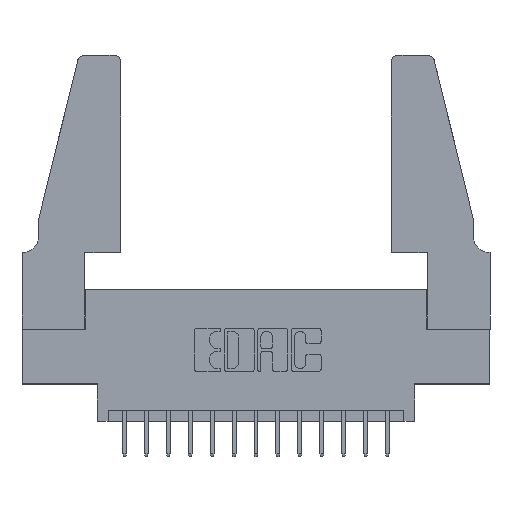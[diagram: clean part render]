
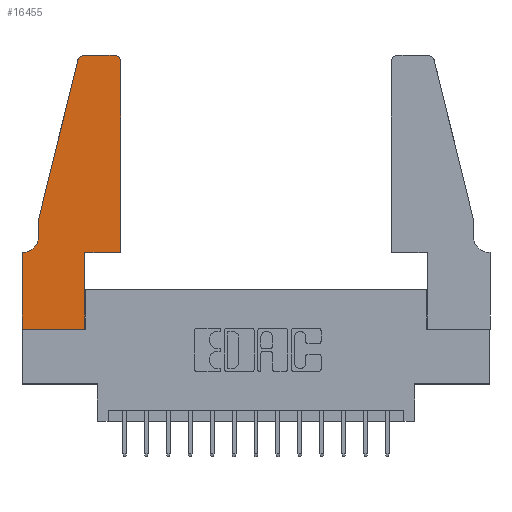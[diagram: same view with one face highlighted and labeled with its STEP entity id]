
A CAD part, top view. The second image highlights one B-rep face of the part: STEP entity #16455.
In plain terms, the highlighted planar face has unit normal (0, 0, 1).
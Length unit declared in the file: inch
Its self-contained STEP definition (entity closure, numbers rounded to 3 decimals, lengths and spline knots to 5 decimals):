
#24 = CARTESIAN_POINT ( 'NONE',  ( 0.0755, 0.5, 0.37 ) ) ;
#61 = CARTESIAN_POINT ( 'NONE',  ( 0.284, 1.25, 0.37 ) ) ;
#495 = ORIENTED_EDGE ( 'NONE', *, *, #12452, .T. ) ;
#755 = CARTESIAN_POINT ( 'NONE',  ( 0.2865, 0., 0.37 ) ) ;
#765 = CARTESIAN_POINT ( 'NONE',  ( 0.0755, 0.5, 0.37 ) ) ;
#875 = VERTEX_POINT ( 'NONE', #9621 ) ;
#919 = VECTOR ( 'NONE', #1364, 39.37008 ) ;
#1268 = ORIENTED_EDGE ( 'NONE', *, *, #7917, .T. ) ;
#1325 = VECTOR ( 'NONE', #1916, 39.37008 ) ;
#1364 = DIRECTION ( 'NONE',  ( -0.239, -0.971, 0. ) ) ;
#1634 = VECTOR ( 'NONE', #3350, 39.37008 ) ;
#1874 = CIRCLE ( 'NONE', #6621, 0.03 ) ;
#1916 = DIRECTION ( 'NONE',  ( 1., 0., 0. ) ) ;
#1967 = CARTESIAN_POINT ( 'NONE',  ( 0., 0., 0.37 ) ) ;
#2182 = ORIENTED_EDGE ( 'NONE', *, *, #4784, .T. ) ;
#2227 = VECTOR ( 'NONE', #13800, 39.37008 ) ;
#2240 = DIRECTION ( 'NONE',  ( 0., 0., 1. ) ) ;
#2303 = VERTEX_POINT ( 'NONE', #6227 ) ;
#2391 = LINE ( 'NONE', #16408, #8820 ) ;
#2397 = CARTESIAN_POINT ( 'NONE',  ( 0.4505, 1.22, 0.37 ) ) ;
#2732 = CARTESIAN_POINT ( 'NONE',  ( 0.4505, 0.35, 0.37 ) ) ;
#2824 = VERTEX_POINT ( 'NONE', #12180 ) ;
#2920 = EDGE_CURVE ( 'NONE', #9655, #12077, #4256, .T. ) ;
#3118 = PLANE ( 'NONE',  #6159 ) ;
#3288 = EDGE_CURVE ( 'NONE', #2824, #10259, #14769, .T. ) ;
#3350 = DIRECTION ( 'NONE',  ( -1., 0., 0. ) ) ;
#3437 = ORIENTED_EDGE ( 'NONE', *, *, #3288, .T. ) ;
#3443 = CARTESIAN_POINT ( 'NONE',  ( 0.0755, 0.35, 0.37 ) ) ;
#3829 = ORIENTED_EDGE ( 'NONE', *, *, #7589, .T. ) ;
#3847 = EDGE_CURVE ( 'NONE', #9854, #9655, #5633, .T. ) ;
#4188 = CARTESIAN_POINT ( 'NONE',  ( 0., 0., 0.37 ) ) ;
#4256 = CIRCLE ( 'NONE', #9482, 0.03 ) ;
#4360 = ORIENTED_EDGE ( 'NONE', *, *, #8823, .T. ) ;
#4362 = DIRECTION ( 'NONE',  ( -1., 0., 0. ) ) ;
#4373 = DIRECTION ( 'NONE',  ( 0., 0., -1. ) ) ;
#4391 = CARTESIAN_POINT ( 'NONE',  ( 0.0055, 0.42, 0.37 ) ) ;
#4414 = CARTESIAN_POINT ( 'NONE',  ( 0., 0.35, 0.37 ) ) ;
#4738 = LINE ( 'NONE', #1967, #1325 ) ;
#4784 = EDGE_CURVE ( 'NONE', #9501, #2303, #5204, .T. ) ;
#5204 = LINE ( 'NONE', #9227, #15298 ) ;
#5311 = EDGE_CURVE ( 'NONE', #6510, #2824, #8772, .T. ) ;
#5583 = EDGE_CURVE ( 'NONE', #16345, #9501, #4738, .T. ) ;
#5633 = LINE ( 'NONE', #13785, #2227 ) ;
#5704 = DIRECTION ( 'NONE',  ( 0., 0., 1. ) ) ;
#6159 = AXIS2_PLACEMENT_3D ( 'NONE', #4414, #5704, #14575 ) ;
#6227 = CARTESIAN_POINT ( 'NONE',  ( 0.2865, 0.35, 0.37 ) ) ;
#6401 = ORIENTED_EDGE ( 'NONE', *, *, #11606, .T. ) ;
#6418 = ORIENTED_EDGE ( 'NONE', *, *, #13967, .T. ) ;
#6510 = VERTEX_POINT ( 'NONE', #14162 ) ;
#6621 = AXIS2_PLACEMENT_3D ( 'NONE', #9895, #2240, #11123 ) ;
#6858 = LINE ( 'NONE', #10483, #8945 ) ;
#7440 = VECTOR ( 'NONE', #13553, 39.37008 ) ;
#7589 = EDGE_CURVE ( 'NONE', #9168, #875, #1874, .T. ) ;
#7593 = DIRECTION ( 'NONE',  ( 1., 0., 0. ) ) ;
#7917 = EDGE_CURVE ( 'NONE', #10259, #16345, #6858, .T. ) ;
#8772 = CIRCLE ( 'NONE', #14871, 0.07 ) ;
#8820 = VECTOR ( 'NONE', #7593, 39.37008 ) ;
#8823 = EDGE_CURVE ( 'NONE', #14303, #6510, #14197, .T. ) ;
#8945 = VECTOR ( 'NONE', #11729, 39.37008 ) ;
#9124 = ORIENTED_EDGE ( 'NONE', *, *, #3847, .T. ) ;
#9168 = VERTEX_POINT ( 'NONE', #61 ) ;
#9227 = CARTESIAN_POINT ( 'NONE',  ( 0.2865, 0.35, 0.37 ) ) ;
#9345 = DIRECTION ( 'NONE',  ( 0., 1., 0. ) ) ;
#9482 = AXIS2_PLACEMENT_3D ( 'NONE', #9746, #9694, #9692 ) ;
#9501 = VERTEX_POINT ( 'NONE', #755 ) ;
#9608 = EDGE_LOOP ( 'NONE', ( #495, #3829, #6418, #4360, #15660, #3437, #1268, #9842, #2182, #6401, #9124, #11259 ) ) ;
#9621 = CARTESIAN_POINT ( 'NONE',  ( 0.25487, 1.22718, 0.37 ) ) ;
#9655 = VERTEX_POINT ( 'NONE', #2397 ) ;
#9664 = FACE_OUTER_BOUND ( 'NONE', #9608, .T. ) ;
#9692 = DIRECTION ( 'NONE',  ( 1., 0., 0. ) ) ;
#9694 = DIRECTION ( 'NONE',  ( 0., 0., 1. ) ) ;
#9746 = CARTESIAN_POINT ( 'NONE',  ( 0.4205, 1.22, 0.37 ) ) ;
#9842 = ORIENTED_EDGE ( 'NONE', *, *, #5583, .T. ) ;
#9854 = VERTEX_POINT ( 'NONE', #2732 ) ;
#9895 = CARTESIAN_POINT ( 'NONE',  ( 0.284, 1.22, 0.37 ) ) ;
#10259 = VERTEX_POINT ( 'NONE', #16111 ) ;
#10483 = CARTESIAN_POINT ( 'NONE',  ( 0., 0., 0.37 ) ) ;
#11092 = LINE ( 'NONE', #24, #919 ) ;
#11123 = DIRECTION ( 'NONE',  ( 1., 0., 0. ) ) ;
#11259 = ORIENTED_EDGE ( 'NONE', *, *, #2920, .T. ) ;
#11606 = EDGE_CURVE ( 'NONE', #2303, #9854, #2391, .T. ) ;
#11729 = DIRECTION ( 'NONE',  ( 0., -1., 0. ) ) ;
#12077 = VERTEX_POINT ( 'NONE', #15265 ) ;
#12117 = VECTOR ( 'NONE', #13509, 39.37008 ) ;
#12180 = CARTESIAN_POINT ( 'NONE',  ( 0.0055, 0.35, 0.37 ) ) ;
#12452 = EDGE_CURVE ( 'NONE', #12077, #9168, #12495, .T. ) ;
#12495 = LINE ( 'NONE', #14761, #12117 ) ;
#13453 = CARTESIAN_POINT ( 'NONE',  ( 0.0755, 0.5, 0.37 ) ) ;
#13509 = DIRECTION ( 'NONE',  ( -1., 0., 0. ) ) ;
#13553 = DIRECTION ( 'NONE',  ( 0., -1., 0. ) ) ;
#13785 = CARTESIAN_POINT ( 'NONE',  ( 0.4505, 0.35, 0.37 ) ) ;
#13800 = DIRECTION ( 'NONE',  ( 0., 1., 0. ) ) ;
#13967 = EDGE_CURVE ( 'NONE', #875, #14303, #11092, .T. ) ;
#14162 = CARTESIAN_POINT ( 'NONE',  ( 0.0755, 0.42, 0.37 ) ) ;
#14197 = LINE ( 'NONE', #765, #7440 ) ;
#14303 = VERTEX_POINT ( 'NONE', #13453 ) ;
#14575 = DIRECTION ( 'NONE',  ( 1., 0., 0. ) ) ;
#14761 = CARTESIAN_POINT ( 'NONE',  ( 0.2605, 1.25, 0.37 ) ) ;
#14769 = LINE ( 'NONE', #3443, #1634 ) ;
#14871 = AXIS2_PLACEMENT_3D ( 'NONE', #4391, #4373, #4362 ) ;
#15265 = CARTESIAN_POINT ( 'NONE',  ( 0.4205, 1.25, 0.37 ) ) ;
#15298 = VECTOR ( 'NONE', #9345, 39.37008 ) ;
#15660 = ORIENTED_EDGE ( 'NONE', *, *, #5311, .T. ) ;
#16111 = CARTESIAN_POINT ( 'NONE',  ( 0., 0.35, 0.37 ) ) ;
#16345 = VERTEX_POINT ( 'NONE', #4188 ) ;
#16408 = CARTESIAN_POINT ( 'NONE',  ( 0.4505, 0.35, 0.37 ) ) ;
#16455 = ADVANCED_FACE ( 'NONE', ( #9664 ), #3118, .T. ) ;
